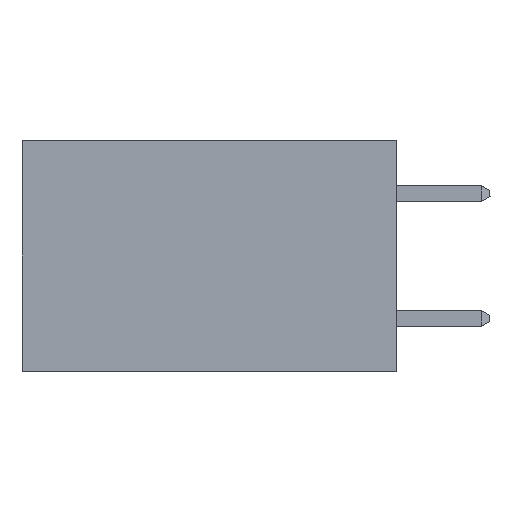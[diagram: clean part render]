
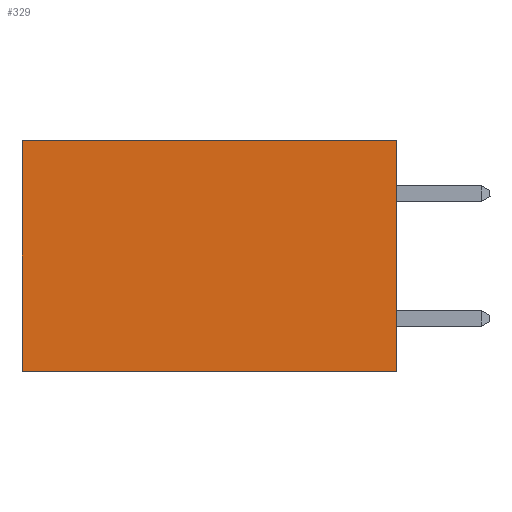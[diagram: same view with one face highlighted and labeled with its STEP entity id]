
A CAD part, left-side view. The second image highlights one B-rep face of the part: STEP entity #329.
In plain terms, the highlighted planar face has unit normal (-1, 0, 0).
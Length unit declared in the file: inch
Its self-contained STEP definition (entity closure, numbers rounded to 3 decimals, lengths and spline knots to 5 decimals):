
#123 = LINE ( 'NONE', #12501, #1198 ) ;
#329 = ADVANCED_FACE ( 'NONE', ( #10394 ), #9489, .F. ) ;
#1111 = VECTOR ( 'NONE', #4383, 39.37008 ) ;
#1198 = VECTOR ( 'NONE', #13889, 39.37008 ) ;
#1545 = VECTOR ( 'NONE', #9547, 39.37008 ) ;
#1576 = CARTESIAN_POINT ( 'NONE',  ( 0.298, 0., -0.37 ) ) ;
#1831 = VERTEX_POINT ( 'NONE', #8203 ) ;
#1876 = EDGE_CURVE ( 'NONE', #6861, #1831, #7088, .T. ) ;
#2475 = CARTESIAN_POINT ( 'NONE',  ( 0.298, 0., 0. ) ) ;
#3038 = LINE ( 'NONE', #1576, #1111 ) ;
#3467 = EDGE_CURVE ( 'NONE', #1831, #14869, #12281, .T. ) ;
#3863 = CARTESIAN_POINT ( 'NONE',  ( 0.298, 0.6, 0. ) ) ;
#3905 = CARTESIAN_POINT ( 'NONE',  ( 0.298, 0., 0. ) ) ;
#4103 = DIRECTION ( 'NONE',  ( 0., 0., -1. ) ) ;
#4383 = DIRECTION ( 'NONE',  ( 0., 1., 0. ) ) ;
#5369 = ORIENTED_EDGE ( 'NONE', *, *, #1876, .T. ) ;
#6758 = DIRECTION ( 'NONE',  ( 0., 0., -1. ) ) ;
#6861 = VERTEX_POINT ( 'NONE', #8074 ) ;
#7088 = LINE ( 'NONE', #2475, #1545 ) ;
#7992 = CARTESIAN_POINT ( 'NONE',  ( 0.298, 0., -0.37 ) ) ;
#8074 = CARTESIAN_POINT ( 'NONE',  ( 0.298, 0., 0. ) ) ;
#8203 = CARTESIAN_POINT ( 'NONE',  ( 0.298, 0.6, 0. ) ) ;
#8838 = EDGE_LOOP ( 'NONE', ( #9726, #9680, #15624, #5369 ) ) ;
#9489 = PLANE ( 'NONE',  #13119 ) ;
#9547 = DIRECTION ( 'NONE',  ( 0., 1., 0. ) ) ;
#9680 = ORIENTED_EDGE ( 'NONE', *, *, #15012, .F. ) ;
#9726 = ORIENTED_EDGE ( 'NONE', *, *, #3467, .T. ) ;
#10330 = CARTESIAN_POINT ( 'NONE',  ( 0.298, 0.6, -0.37 ) ) ;
#10394 = FACE_OUTER_BOUND ( 'NONE', #8838, .T. ) ;
#12281 = LINE ( 'NONE', #3863, #15526 ) ;
#12501 = CARTESIAN_POINT ( 'NONE',  ( 0.298, 0., 0. ) ) ;
#13119 = AXIS2_PLACEMENT_3D ( 'NONE', #3905, #15113, #6758 ) ;
#13889 = DIRECTION ( 'NONE',  ( 0., 0., -1. ) ) ;
#14869 = VERTEX_POINT ( 'NONE', #10330 ) ;
#15012 = EDGE_CURVE ( 'NONE', #16686, #14869, #3038, .T. ) ;
#15113 = DIRECTION ( 'NONE',  ( 1., 0., 0. ) ) ;
#15526 = VECTOR ( 'NONE', #4103, 39.37008 ) ;
#15624 = ORIENTED_EDGE ( 'NONE', *, *, #16280, .F. ) ;
#16280 = EDGE_CURVE ( 'NONE', #6861, #16686, #123, .T. ) ;
#16686 = VERTEX_POINT ( 'NONE', #7992 ) ;
